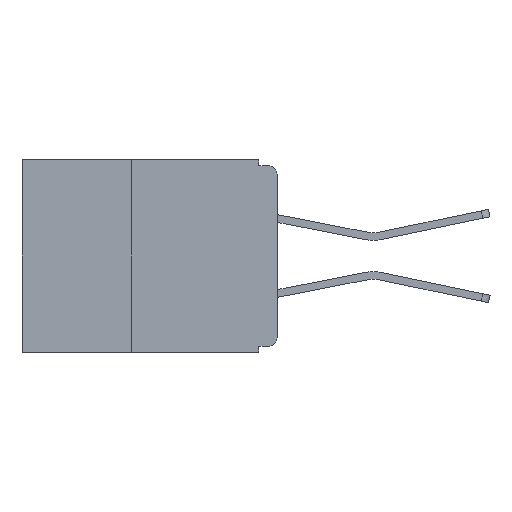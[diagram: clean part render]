
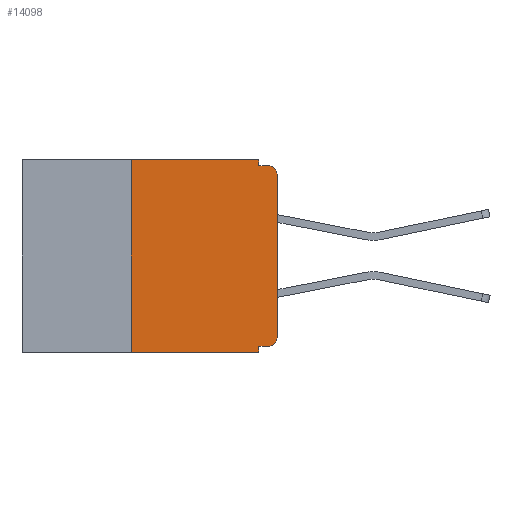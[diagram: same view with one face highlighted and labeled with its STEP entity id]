
A CAD part, left-side view. The second image highlights one B-rep face of the part: STEP entity #14098.
In plain terms, the highlighted planar face has unit normal (-1, 0, 0).
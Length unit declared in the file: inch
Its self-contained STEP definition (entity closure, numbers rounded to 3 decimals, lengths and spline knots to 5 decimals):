
#406 = ORIENTED_EDGE ( 'NONE', *, *, #17950, .F. ) ;
#775 = CARTESIAN_POINT ( 'NONE',  ( 0., 0.25, 0. ) ) ;
#1155 = VERTEX_POINT ( 'NONE', #775 ) ;
#1366 = ORIENTED_EDGE ( 'NONE', *, *, #1641, .T. ) ;
#1641 = EDGE_CURVE ( 'NONE', #17977, #12571, #2022, .T. ) ;
#1713 = DIRECTION ( 'NONE',  ( 0., 1., 0. ) ) ;
#2022 = LINE ( 'NONE', #12627, #12973 ) ;
#2220 = CARTESIAN_POINT ( 'NONE',  ( 0., 0.015, -0.32 ) ) ;
#2226 = EDGE_CURVE ( 'NONE', #19813, #14879, #19714, .T. ) ;
#2354 = CARTESIAN_POINT ( 'NONE',  ( 0., 0.437, 0. ) ) ;
#2982 = CIRCLE ( 'NONE', #19243, 0.015 ) ;
#3041 = VERTEX_POINT ( 'NONE', #9204 ) ;
#3124 = LINE ( 'NONE', #14296, #9461 ) ;
#3148 = CIRCLE ( 'NONE', #14427, 0.015 ) ;
#3198 = AXIS2_PLACEMENT_3D ( 'NONE', #2354, #14803, #5520 ) ;
#3224 = VECTOR ( 'NONE', #1713, 39.37008 ) ;
#3540 = CARTESIAN_POINT ( 'NONE',  ( 0., 0.437, 0. ) ) ;
#3639 = ORIENTED_EDGE ( 'NONE', *, *, #18483, .T. ) ;
#4019 = CARTESIAN_POINT ( 'NONE',  ( 0., 0., -0.01 ) ) ;
#4604 = EDGE_LOOP ( 'NONE', ( #1366, #7748, #15028, #15265, #6515, #406, #3639, #15070, #10434, #9952 ) ) ;
#5248 = CARTESIAN_POINT ( 'NONE',  ( 0., 0.031, -0.33 ) ) ;
#5520 = DIRECTION ( 'NONE',  ( 0., 0., -1. ) ) ;
#5835 = CARTESIAN_POINT ( 'NONE',  ( 0., 0.25, -0.33 ) ) ;
#6364 = VERTEX_POINT ( 'NONE', #13239 ) ;
#6515 = ORIENTED_EDGE ( 'NONE', *, *, #18726, .F. ) ;
#6816 = DIRECTION ( 'NONE',  ( 0., 0., -1. ) ) ;
#7021 = VECTOR ( 'NONE', #6816, 39.37008 ) ;
#7247 = DIRECTION ( 'NONE',  ( -1., 0., 0. ) ) ;
#7473 = VECTOR ( 'NONE', #13876, 39.37008 ) ;
#7605 = DIRECTION ( 'NONE',  ( -1., 0., 0. ) ) ;
#7709 = VECTOR ( 'NONE', #12837, 39.37008 ) ;
#7748 = ORIENTED_EDGE ( 'NONE', *, *, #8956, .T. ) ;
#8097 = DIRECTION ( 'NONE',  ( 0., 0., 1. ) ) ;
#8208 = CARTESIAN_POINT ( 'NONE',  ( 0., 0.031, -0.33 ) ) ;
#8756 = VERTEX_POINT ( 'NONE', #8208 ) ;
#8956 = EDGE_CURVE ( 'NONE', #12571, #11468, #2982, .T. ) ;
#9204 = CARTESIAN_POINT ( 'NONE',  ( 0., 0.031, -0.01 ) ) ;
#9212 = CARTESIAN_POINT ( 'NONE',  ( 0., 0.437, -0.33 ) ) ;
#9447 = VECTOR ( 'NONE', #15465, 39.37008 ) ;
#9461 = VECTOR ( 'NONE', #15885, 39.37008 ) ;
#9952 = ORIENTED_EDGE ( 'NONE', *, *, #16288, .T. ) ;
#10100 = PLANE ( 'NONE',  #3198 ) ;
#10413 = CARTESIAN_POINT ( 'NONE',  ( 0., 0.031, -0.32 ) ) ;
#10434 = ORIENTED_EDGE ( 'NONE', *, *, #2226, .F. ) ;
#10593 = CARTESIAN_POINT ( 'NONE',  ( 0., 0., -0.025 ) ) ;
#10756 = CARTESIAN_POINT ( 'NONE',  ( 0., 0.25, -0.33 ) ) ;
#11123 = LINE ( 'NONE', #4019, #14301 ) ;
#11468 = VERTEX_POINT ( 'NONE', #15697 ) ;
#11553 = LINE ( 'NONE', #9212, #7473 ) ;
#11590 = LINE ( 'NONE', #5248, #7021 ) ;
#11794 = LINE ( 'NONE', #3540, #7709 ) ;
#11896 = VERTEX_POINT ( 'NONE', #5835 ) ;
#11971 = FACE_OUTER_BOUND ( 'NONE', #4604, .T. ) ;
#12189 = EDGE_CURVE ( 'NONE', #6364, #3041, #3124, .T. ) ;
#12414 = EDGE_CURVE ( 'NONE', #3041, #11468, #11123, .T. ) ;
#12571 = VERTEX_POINT ( 'NONE', #10593 ) ;
#12627 = CARTESIAN_POINT ( 'NONE',  ( 0., 0., 0. ) ) ;
#12837 = DIRECTION ( 'NONE',  ( 0., -1., 0. ) ) ;
#12973 = VECTOR ( 'NONE', #8097, 39.37008 ) ;
#13239 = CARTESIAN_POINT ( 'NONE',  ( 0., 0.031, 0. ) ) ;
#13333 = DIRECTION ( 'NONE',  ( 0., -1., 0. ) ) ;
#13555 = LINE ( 'NONE', #10756, #9447 ) ;
#13876 = DIRECTION ( 'NONE',  ( 0., -1., 0. ) ) ;
#14098 = ADVANCED_FACE ( 'NONE', ( #11971 ), #10100, .F. ) ;
#14296 = CARTESIAN_POINT ( 'NONE',  ( 0., 0.031, 0. ) ) ;
#14301 = VECTOR ( 'NONE', #13333, 39.37008 ) ;
#14427 = AXIS2_PLACEMENT_3D ( 'NONE', #16911, #7605, #18434 ) ;
#14803 = DIRECTION ( 'NONE',  ( 1., 0., 0. ) ) ;
#14879 = VERTEX_POINT ( 'NONE', #10413 ) ;
#15028 = ORIENTED_EDGE ( 'NONE', *, *, #12414, .F. ) ;
#15070 = ORIENTED_EDGE ( 'NONE', *, *, #16961, .F. ) ;
#15265 = ORIENTED_EDGE ( 'NONE', *, *, #12189, .F. ) ;
#15465 = DIRECTION ( 'NONE',  ( 0., 0., 1. ) ) ;
#15697 = CARTESIAN_POINT ( 'NONE',  ( 0., 0.015, -0.01 ) ) ;
#15712 = CARTESIAN_POINT ( 'NONE',  ( 0., 0., -0.32 ) ) ;
#15885 = DIRECTION ( 'NONE',  ( 0., 0., -1. ) ) ;
#16288 = EDGE_CURVE ( 'NONE', #19813, #17977, #3148, .T. ) ;
#16571 = CARTESIAN_POINT ( 'NONE',  ( 0., 0.015, -0.025 ) ) ;
#16911 = CARTESIAN_POINT ( 'NONE',  ( 0., 0.015, -0.305 ) ) ;
#16961 = EDGE_CURVE ( 'NONE', #14879, #8756, #11590, .T. ) ;
#17037 = CARTESIAN_POINT ( 'NONE',  ( 0., 0., -0.305 ) ) ;
#17950 = EDGE_CURVE ( 'NONE', #11896, #1155, #13555, .T. ) ;
#17977 = VERTEX_POINT ( 'NONE', #17037 ) ;
#18096 = DIRECTION ( 'NONE',  ( 0., 0., -1. ) ) ;
#18434 = DIRECTION ( 'NONE',  ( 0., 0., -1. ) ) ;
#18483 = EDGE_CURVE ( 'NONE', #11896, #8756, #11553, .T. ) ;
#18726 = EDGE_CURVE ( 'NONE', #1155, #6364, #11794, .T. ) ;
#19243 = AXIS2_PLACEMENT_3D ( 'NONE', #16571, #7247, #18096 ) ;
#19714 = LINE ( 'NONE', #15712, #3224 ) ;
#19813 = VERTEX_POINT ( 'NONE', #2220 ) ;
